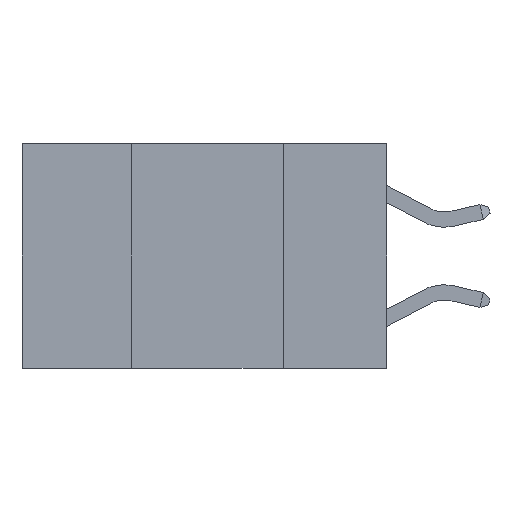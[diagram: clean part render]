
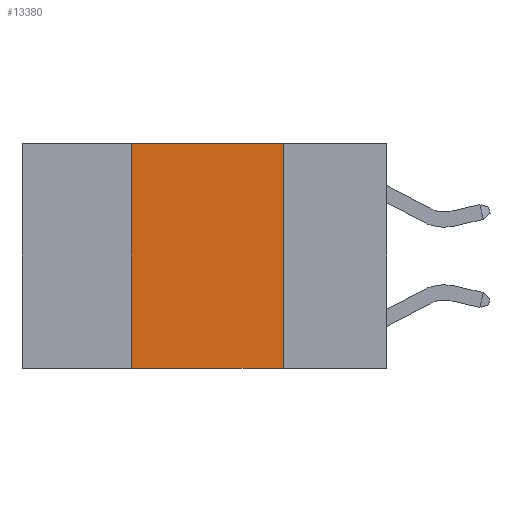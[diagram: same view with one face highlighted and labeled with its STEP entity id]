
A CAD part, left-side view. The second image highlights one B-rep face of the part: STEP entity #13380.
In plain terms, the highlighted planar face has unit normal (-1, 0, 0).
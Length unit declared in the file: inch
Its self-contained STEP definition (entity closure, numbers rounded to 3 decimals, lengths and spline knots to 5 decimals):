
#56 = DIRECTION ( 'NONE',  ( 0., -1., 0. ) ) ;
#588 = CARTESIAN_POINT ( 'NONE',  ( 0., 0.17, -0.37 ) ) ;
#700 = CARTESIAN_POINT ( 'NONE',  ( 0., 0.6, 0. ) ) ;
#1190 = ORIENTED_EDGE ( 'NONE', *, *, #7804, .F. ) ;
#1460 = ORIENTED_EDGE ( 'NONE', *, *, #2661, .F. ) ;
#1513 = VERTEX_POINT ( 'NONE', #12757 ) ;
#2002 = CARTESIAN_POINT ( 'NONE',  ( 0., 0.17, 0. ) ) ;
#2033 = VERTEX_POINT ( 'NONE', #2266 ) ;
#2266 = CARTESIAN_POINT ( 'NONE',  ( 0., 0.42, 0. ) ) ;
#2431 = EDGE_CURVE ( 'NONE', #12913, #2033, #12418, .T. ) ;
#2661 = EDGE_CURVE ( 'NONE', #1513, #4944, #7310, .T. ) ;
#3299 = VECTOR ( 'NONE', #13120, 39.37008 ) ;
#3712 = EDGE_CURVE ( 'NONE', #12913, #4944, #8635, .T. ) ;
#4105 = DIRECTION ( 'NONE',  ( 1., 0., 0. ) ) ;
#4944 = VERTEX_POINT ( 'NONE', #588 ) ;
#7310 = LINE ( 'NONE', #2002, #13282 ) ;
#7667 = DIRECTION ( 'NONE',  ( 0., -1., 0. ) ) ;
#7804 = EDGE_CURVE ( 'NONE', #2033, #1513, #7961, .T. ) ;
#7961 = LINE ( 'NONE', #700, #9930 ) ;
#8635 = LINE ( 'NONE', #9386, #11243 ) ;
#8745 = CARTESIAN_POINT ( 'NONE',  ( 0., 0.6, 0. ) ) ;
#9268 = ORIENTED_EDGE ( 'NONE', *, *, #3712, .T. ) ;
#9386 = CARTESIAN_POINT ( 'NONE',  ( 0., 0.6, -0.37 ) ) ;
#9589 = FACE_OUTER_BOUND ( 'NONE', #10009, .T. ) ;
#9930 = VECTOR ( 'NONE', #7667, 39.37008 ) ;
#10009 = EDGE_LOOP ( 'NONE', ( #1460, #1190, #14048, #9268 ) ) ;
#10984 = PLANE ( 'NONE',  #11622 ) ;
#11188 = DIRECTION ( 'NONE',  ( 0., 0., -1. ) ) ;
#11243 = VECTOR ( 'NONE', #56, 39.37008 ) ;
#11622 = AXIS2_PLACEMENT_3D ( 'NONE', #8745, #4105, #12096 ) ;
#12022 = CARTESIAN_POINT ( 'NONE',  ( 0., 0.42, 0. ) ) ;
#12096 = DIRECTION ( 'NONE',  ( 0., 0., -1. ) ) ;
#12418 = LINE ( 'NONE', #12022, #3299 ) ;
#12729 = CARTESIAN_POINT ( 'NONE',  ( 0., 0.42, -0.37 ) ) ;
#12757 = CARTESIAN_POINT ( 'NONE',  ( 0., 0.17, 0. ) ) ;
#12913 = VERTEX_POINT ( 'NONE', #12729 ) ;
#13120 = DIRECTION ( 'NONE',  ( 0., 0., 1. ) ) ;
#13282 = VECTOR ( 'NONE', #11188, 39.37008 ) ;
#13380 = ADVANCED_FACE ( 'NONE', ( #9589 ), #10984, .F. ) ;
#14048 = ORIENTED_EDGE ( 'NONE', *, *, #2431, .F. ) ;
